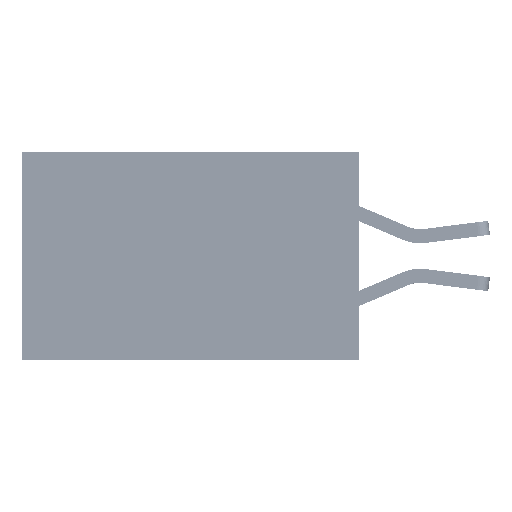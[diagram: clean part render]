
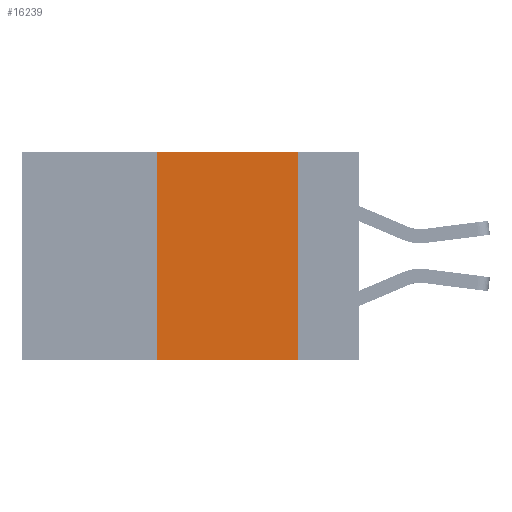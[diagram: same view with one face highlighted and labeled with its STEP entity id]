
A CAD part, left-side view. The second image highlights one B-rep face of the part: STEP entity #16239.
In plain terms, the highlighted planar face has unit normal (-1, 0, 0).
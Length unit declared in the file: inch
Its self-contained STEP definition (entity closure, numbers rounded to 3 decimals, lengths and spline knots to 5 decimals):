
#40 = AXIS2_PLACEMENT_3D ( 'NONE', #16459, #31341, #31152 ) ;
#168 = DIRECTION ( 'NONE',  ( 0., -1., 0. ) ) ;
#2809 = CARTESIAN_POINT ( 'NONE',  ( 0., 0.6, -0.37 ) ) ;
#3360 = CARTESIAN_POINT ( 'NONE',  ( 0., 0.36, 0. ) ) ;
#3437 = VECTOR ( 'NONE', #17459, 39.37008 ) ;
#3593 = CARTESIAN_POINT ( 'NONE',  ( 0., 0.6, 0. ) ) ;
#5818 = EDGE_CURVE ( 'NONE', #19130, #16322, #15066, .T. ) ;
#7181 = PLANE ( 'NONE',  #40 ) ;
#10998 = LINE ( 'NONE', #23668, #3437 ) ;
#11565 = VERTEX_POINT ( 'NONE', #34993 ) ;
#14346 = EDGE_CURVE ( 'NONE', #11565, #22636, #24533, .T. ) ;
#15066 = LINE ( 'NONE', #3593, #38673 ) ;
#16239 = ADVANCED_FACE ( 'NONE', ( #18879 ), #7181, .F. ) ;
#16322 = VERTEX_POINT ( 'NONE', #28534 ) ;
#16459 = CARTESIAN_POINT ( 'NONE',  ( 0., 0.6, 0. ) ) ;
#17459 = DIRECTION ( 'NONE',  ( 0., 0., -1. ) ) ;
#17495 = CARTESIAN_POINT ( 'NONE',  ( 0., 0.36, 0. ) ) ;
#18007 = ORIENTED_EDGE ( 'NONE', *, *, #26000, .F. ) ;
#18879 = FACE_OUTER_BOUND ( 'NONE', #35992, .T. ) ;
#19130 = VERTEX_POINT ( 'NONE', #3360 ) ;
#20418 = VECTOR ( 'NONE', #27898, 39.37008 ) ;
#21552 = CARTESIAN_POINT ( 'NONE',  ( 0., 0.11, -0.37 ) ) ;
#21895 = ORIENTED_EDGE ( 'NONE', *, *, #14346, .T. ) ;
#22636 = VERTEX_POINT ( 'NONE', #21552 ) ;
#23668 = CARTESIAN_POINT ( 'NONE',  ( 0., 0.11, 0. ) ) ;
#24533 = LINE ( 'NONE', #2809, #37195 ) ;
#24609 = ORIENTED_EDGE ( 'NONE', *, *, #5818, .F. ) ;
#26000 = EDGE_CURVE ( 'NONE', #16322, #22636, #10998, .T. ) ;
#26983 = DIRECTION ( 'NONE',  ( 0., -1., 0. ) ) ;
#27898 = DIRECTION ( 'NONE',  ( 0., 0., 1. ) ) ;
#28534 = CARTESIAN_POINT ( 'NONE',  ( 0., 0.11, 0. ) ) ;
#31152 = DIRECTION ( 'NONE',  ( 0., 0., -1. ) ) ;
#31341 = DIRECTION ( 'NONE',  ( 1., 0., 0. ) ) ;
#33830 = ORIENTED_EDGE ( 'NONE', *, *, #35377, .F. ) ;
#33909 = LINE ( 'NONE', #17495, #20418 ) ;
#34993 = CARTESIAN_POINT ( 'NONE',  ( 0., 0.36, -0.37 ) ) ;
#35377 = EDGE_CURVE ( 'NONE', #11565, #19130, #33909, .T. ) ;
#35992 = EDGE_LOOP ( 'NONE', ( #18007, #24609, #33830, #21895 ) ) ;
#37195 = VECTOR ( 'NONE', #26983, 39.37008 ) ;
#38673 = VECTOR ( 'NONE', #168, 39.37008 ) ;
